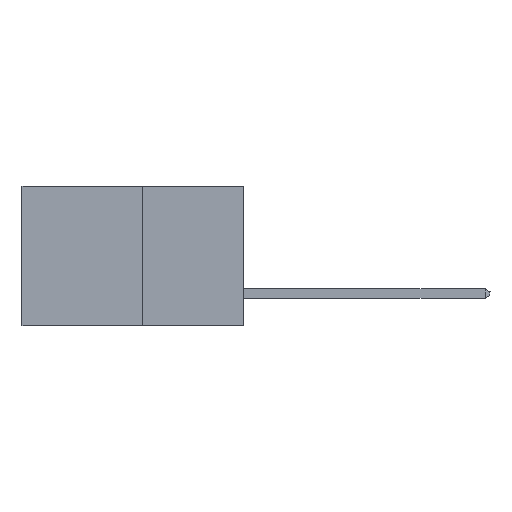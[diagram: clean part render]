
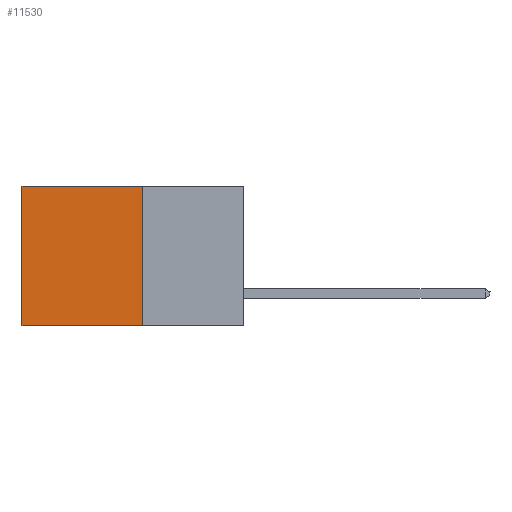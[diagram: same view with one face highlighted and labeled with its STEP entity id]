
A CAD part, left-side view. The second image highlights one B-rep face of the part: STEP entity #11530.
In plain terms, the highlighted planar face has unit normal (-1, 0, 0).
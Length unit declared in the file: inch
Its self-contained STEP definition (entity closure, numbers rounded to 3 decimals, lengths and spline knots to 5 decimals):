
#43 = EDGE_CURVE ( 'NONE', #16297, #10389, #3168, .T. ) ;
#177 = DIRECTION ( 'NONE',  ( 0., 1., 0. ) ) ;
#1396 = PLANE ( 'NONE',  #8256 ) ;
#2052 = EDGE_CURVE ( 'NONE', #10389, #6989, #15637, .T. ) ;
#2869 = DIRECTION ( 'NONE',  ( 1., 0., 0. ) ) ;
#3168 = LINE ( 'NONE', #9527, #9693 ) ;
#4772 = VERTEX_POINT ( 'NONE', #9581 ) ;
#5087 = EDGE_CURVE ( 'NONE', #16297, #4772, #13911, .T. ) ;
#5488 = LINE ( 'NONE', #11046, #15586 ) ;
#5854 = CARTESIAN_POINT ( 'NONE',  ( 0.277, 0.27, 0. ) ) ;
#6073 = DIRECTION ( 'NONE',  ( 0., 1., 0. ) ) ;
#6793 = VECTOR ( 'NONE', #177, 39.37008 ) ;
#6989 = VERTEX_POINT ( 'NONE', #10409 ) ;
#7073 = VECTOR ( 'NONE', #6073, 39.37008 ) ;
#7608 = CARTESIAN_POINT ( 'NONE',  ( 0.277, 0.27, -0.37 ) ) ;
#8256 = AXIS2_PLACEMENT_3D ( 'NONE', #13026, #2869, #11844 ) ;
#8837 = ORIENTED_EDGE ( 'NONE', *, *, #5087, .T. ) ;
#8893 = ORIENTED_EDGE ( 'NONE', *, *, #43, .F. ) ;
#9030 = ORIENTED_EDGE ( 'NONE', *, *, #2052, .F. ) ;
#9289 = ORIENTED_EDGE ( 'NONE', *, *, #13211, .T. ) ;
#9527 = CARTESIAN_POINT ( 'NONE',  ( 0.277, 0.27, -0.37 ) ) ;
#9581 = CARTESIAN_POINT ( 'NONE',  ( 0.277, 0.59, 0. ) ) ;
#9693 = VECTOR ( 'NONE', #12639, 39.37008 ) ;
#9791 = EDGE_LOOP ( 'NONE', ( #9289, #9030, #8893, #8837 ) ) ;
#10389 = VERTEX_POINT ( 'NONE', #7608 ) ;
#10409 = CARTESIAN_POINT ( 'NONE',  ( 0.277, 0.59, -0.37 ) ) ;
#11046 = CARTESIAN_POINT ( 'NONE',  ( 0.277, 0.59, -0.37 ) ) ;
#11530 = ADVANCED_FACE ( 'NONE', ( #12327 ), #1396, .F. ) ;
#11844 = DIRECTION ( 'NONE',  ( 0., 0., -1. ) ) ;
#12007 = CARTESIAN_POINT ( 'NONE',  ( 0.277, 0.27, 0. ) ) ;
#12294 = DIRECTION ( 'NONE',  ( 0., 0., -1. ) ) ;
#12327 = FACE_OUTER_BOUND ( 'NONE', #9791, .T. ) ;
#12401 = CARTESIAN_POINT ( 'NONE',  ( 0.277, 0.27, -0.37 ) ) ;
#12639 = DIRECTION ( 'NONE',  ( 0., 0., -1. ) ) ;
#13026 = CARTESIAN_POINT ( 'NONE',  ( 0.277, 0.27, -0.37 ) ) ;
#13211 = EDGE_CURVE ( 'NONE', #4772, #6989, #5488, .T. ) ;
#13911 = LINE ( 'NONE', #5854, #7073 ) ;
#15586 = VECTOR ( 'NONE', #12294, 39.37008 ) ;
#15637 = LINE ( 'NONE', #12401, #6793 ) ;
#16297 = VERTEX_POINT ( 'NONE', #12007 ) ;
